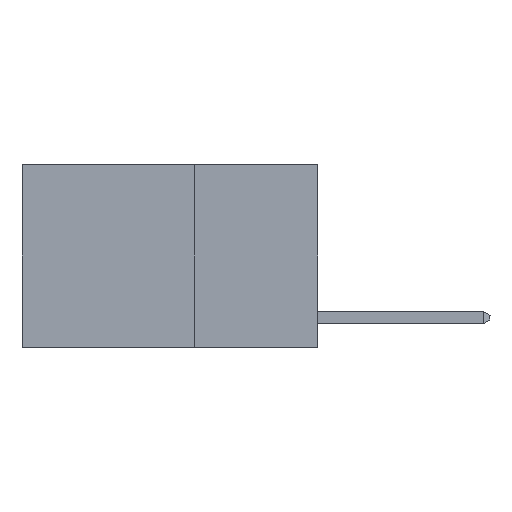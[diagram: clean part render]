
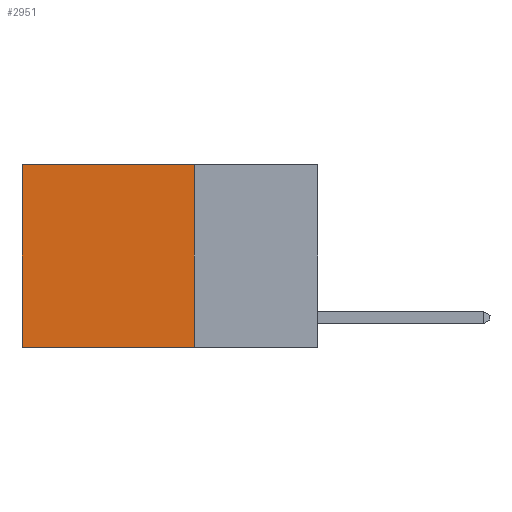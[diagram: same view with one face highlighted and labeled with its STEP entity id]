
A CAD part, left-side view. The second image highlights one B-rep face of the part: STEP entity #2951.
In plain terms, the highlighted planar face has unit normal (-1, 0, 0).
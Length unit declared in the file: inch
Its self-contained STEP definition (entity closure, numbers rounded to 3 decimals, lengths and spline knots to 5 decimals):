
#1450 = CARTESIAN_POINT ( 'NONE',  ( 0.2625, 0.6, -0.37 ) ) ;
#1658 = CARTESIAN_POINT ( 'NONE',  ( 0.2625, 0.25, 0. ) ) ;
#1877 = CARTESIAN_POINT ( 'NONE',  ( 0.2625, 0.25, -0.37 ) ) ;
#1979 = CARTESIAN_POINT ( 'NONE',  ( 0.2625, 0.25, 0. ) ) ;
#2231 = VERTEX_POINT ( 'NONE', #1450 ) ;
#2951 = ADVANCED_FACE ( 'NONE', ( #12276 ), #2984, .F. ) ;
#2984 = PLANE ( 'NONE',  #7676 ) ;
#3124 = VECTOR ( 'NONE', #8474, 39.37008 ) ;
#4290 = DIRECTION ( 'NONE',  ( 1., 0., 0. ) ) ;
#4481 = ORIENTED_EDGE ( 'NONE', *, *, #14332, .F. ) ;
#5592 = LINE ( 'NONE', #7557, #11320 ) ;
#6390 = CARTESIAN_POINT ( 'NONE',  ( 0.2625, 0.6, 0. ) ) ;
#6574 = EDGE_CURVE ( 'NONE', #12790, #2231, #9825, .T. ) ;
#7187 = VERTEX_POINT ( 'NONE', #1979 ) ;
#7557 = CARTESIAN_POINT ( 'NONE',  ( 0.2625, 0.25, -0.37 ) ) ;
#7676 = AXIS2_PLACEMENT_3D ( 'NONE', #1658, #4290, #12910 ) ;
#7831 = LINE ( 'NONE', #9043, #13848 ) ;
#8474 = DIRECTION ( 'NONE',  ( 0., 0., -1. ) ) ;
#8703 = ORIENTED_EDGE ( 'NONE', *, *, #16063, .T. ) ;
#9043 = CARTESIAN_POINT ( 'NONE',  ( 0.2625, 0.25, 0. ) ) ;
#9310 = VERTEX_POINT ( 'NONE', #1877 ) ;
#9825 = LINE ( 'NONE', #14448, #3124 ) ;
#11242 = CARTESIAN_POINT ( 'NONE',  ( 0.2625, 0.25, 0. ) ) ;
#11320 = VECTOR ( 'NONE', #14678, 39.37008 ) ;
#11472 = EDGE_CURVE ( 'NONE', #9310, #2231, #5592, .T. ) ;
#11550 = VECTOR ( 'NONE', #13639, 39.37008 ) ;
#11767 = ORIENTED_EDGE ( 'NONE', *, *, #6574, .T. ) ;
#12276 = FACE_OUTER_BOUND ( 'NONE', #15462, .T. ) ;
#12790 = VERTEX_POINT ( 'NONE', #6390 ) ;
#12910 = DIRECTION ( 'NONE',  ( 0., 0., -1. ) ) ;
#13639 = DIRECTION ( 'NONE',  ( 0., 1., 0. ) ) ;
#13848 = VECTOR ( 'NONE', #15005, 39.37008 ) ;
#14332 = EDGE_CURVE ( 'NONE', #7187, #9310, #7831, .T. ) ;
#14448 = CARTESIAN_POINT ( 'NONE',  ( 0.2625, 0.6, 0. ) ) ;
#14644 = ORIENTED_EDGE ( 'NONE', *, *, #11472, .F. ) ;
#14678 = DIRECTION ( 'NONE',  ( 0., 1., 0. ) ) ;
#14704 = LINE ( 'NONE', #11242, #11550 ) ;
#15005 = DIRECTION ( 'NONE',  ( 0., 0., -1. ) ) ;
#15462 = EDGE_LOOP ( 'NONE', ( #11767, #14644, #4481, #8703 ) ) ;
#16063 = EDGE_CURVE ( 'NONE', #7187, #12790, #14704, .T. ) ;
